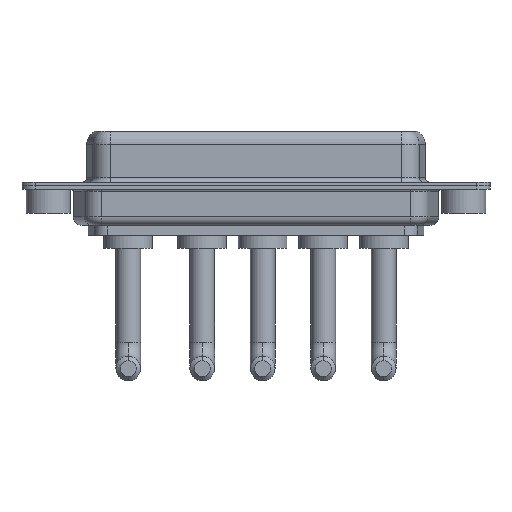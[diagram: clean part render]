
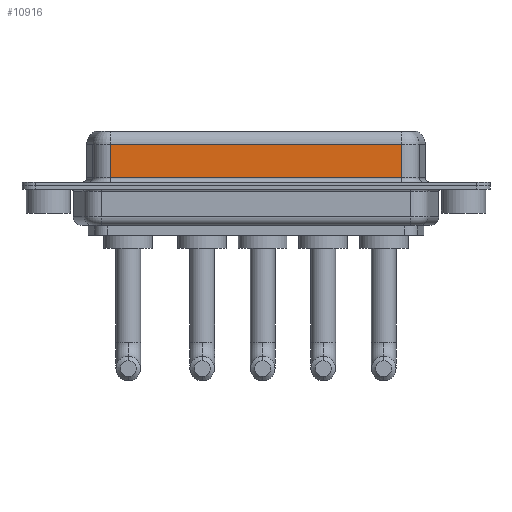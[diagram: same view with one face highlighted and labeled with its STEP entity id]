
A CAD part, front view. The second image highlights one B-rep face of the part: STEP entity #10916.
In plain terms, the highlighted planar face has unit normal (0, -1, 0).
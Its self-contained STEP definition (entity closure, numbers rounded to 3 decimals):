
#323 = VERTEX_POINT ( 'NONE', #2565 ) ;
#388 = DIRECTION ( 'NONE',  ( -1., 0., 0. ) ) ;
#492 = CARTESIAN_POINT ( 'NONE',  ( 40.037, -3.95, 0.9 ) ) ;
#582 = CARTESIAN_POINT ( 'NONE',  ( 40.037, -3.95, 4.65 ) ) ;
#1761 = CARTESIAN_POINT ( 'NONE',  ( 7.013, -3.95, 4.65 ) ) ;
#2331 = ORIENTED_EDGE ( 'NONE', *, *, #6808, .T. ) ;
#2565 = CARTESIAN_POINT ( 'NONE',  ( 7.013, -3.95, 0.9 ) ) ;
#2819 = EDGE_LOOP ( 'NONE', ( #11118, #2331, #3278, #10480 ) ) ;
#3278 = ORIENTED_EDGE ( 'NONE', *, *, #3879, .T. ) ;
#3820 = DIRECTION ( 'NONE',  ( 1., 0., 0. ) ) ;
#3879 = EDGE_CURVE ( 'NONE', #10134, #323, #8078, .T. ) ;
#4053 = VECTOR ( 'NONE', #3820, 1000. ) ;
#5524 = CARTESIAN_POINT ( 'NONE',  ( 40.037, -3.95, 4.65 ) ) ;
#5546 = CARTESIAN_POINT ( 'NONE',  ( 40.037, -3.95, 6.4 ) ) ;
#6239 = VERTEX_POINT ( 'NONE', #492 ) ;
#6444 = DIRECTION ( 'NONE',  ( 0., 1., 0. ) ) ;
#6808 = EDGE_CURVE ( 'NONE', #8124, #10134, #12346, .T. ) ;
#7042 = DIRECTION ( 'NONE',  ( 0., 0., -1. ) ) ;
#7342 = FACE_OUTER_BOUND ( 'NONE', #2819, .T. ) ;
#7822 = CARTESIAN_POINT ( 'NONE',  ( 7.013, -3.95, 6.4 ) ) ;
#8078 = LINE ( 'NONE', #7822, #8918 ) ;
#8124 = VERTEX_POINT ( 'NONE', #5524 ) ;
#8456 = VECTOR ( 'NONE', #10803, 1000. ) ;
#8737 = LINE ( 'NONE', #12606, #4053 ) ;
#8918 = VECTOR ( 'NONE', #7042, 1000. ) ;
#9148 = EDGE_CURVE ( 'NONE', #8124, #6239, #11641, .T. ) ;
#10134 = VERTEX_POINT ( 'NONE', #1761 ) ;
#10267 = DIRECTION ( 'NONE',  ( 0., 0., 1. ) ) ;
#10333 = PLANE ( 'NONE',  #12349 ) ;
#10480 = ORIENTED_EDGE ( 'NONE', *, *, #12728, .T. ) ;
#10803 = DIRECTION ( 'NONE',  ( 0., 0., -1. ) ) ;
#10916 = ADVANCED_FACE ( 'NONE', ( #7342 ), #10333, .F. ) ;
#10977 = VECTOR ( 'NONE', #388, 1000. ) ;
#11118 = ORIENTED_EDGE ( 'NONE', *, *, #9148, .F. ) ;
#11641 = LINE ( 'NONE', #12594, #8456 ) ;
#12346 = LINE ( 'NONE', #582, #10977 ) ;
#12349 = AXIS2_PLACEMENT_3D ( 'NONE', #5546, #6444, #10267 ) ;
#12594 = CARTESIAN_POINT ( 'NONE',  ( 40.037, -3.95, 6.4 ) ) ;
#12606 = CARTESIAN_POINT ( 'NONE',  ( 40.037, -3.95, 0.9 ) ) ;
#12728 = EDGE_CURVE ( 'NONE', #323, #6239, #8737, .T. ) ;
